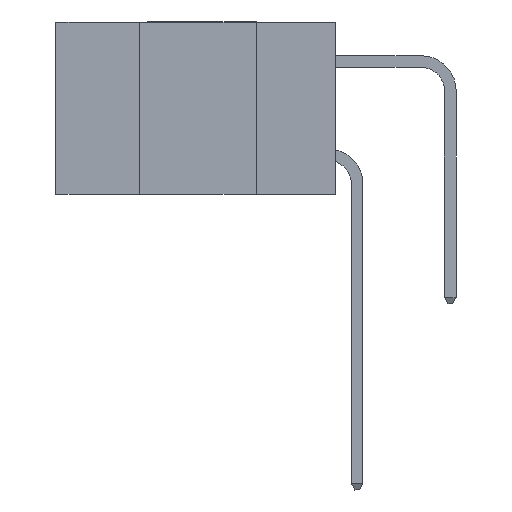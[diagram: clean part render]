
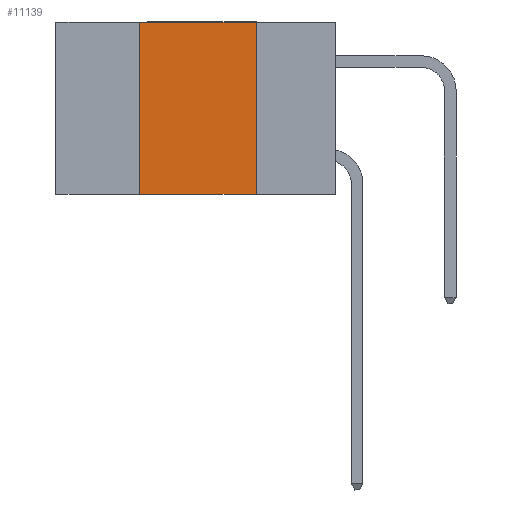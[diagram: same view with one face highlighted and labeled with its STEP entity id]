
A CAD part, left-side view. The second image highlights one B-rep face of the part: STEP entity #11139.
In plain terms, the highlighted planar face has unit normal (-1, 0, 0).
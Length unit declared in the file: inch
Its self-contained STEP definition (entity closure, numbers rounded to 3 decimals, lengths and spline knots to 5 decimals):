
#171 = ORIENTED_EDGE ( 'NONE', *, *, #3334, .F. ) ;
#445 = DIRECTION ( 'NONE',  ( 0., 0., 1. ) ) ;
#1408 = CARTESIAN_POINT ( 'NONE',  ( 0., 0.6, 0. ) ) ;
#2060 = LINE ( 'NONE', #5218, #6798 ) ;
#2243 = LINE ( 'NONE', #3809, #11266 ) ;
#2453 = DIRECTION ( 'NONE',  ( 1., 0., 0. ) ) ;
#2928 = DIRECTION ( 'NONE',  ( 0., -1., 0. ) ) ;
#3334 = EDGE_CURVE ( 'NONE', #9514, #6321, #7796, .T. ) ;
#3809 = CARTESIAN_POINT ( 'NONE',  ( 0., 0.6, -0.37 ) ) ;
#4106 = FACE_OUTER_BOUND ( 'NONE', #6599, .T. ) ;
#4191 = VERTEX_POINT ( 'NONE', #8564 ) ;
#4401 = ORIENTED_EDGE ( 'NONE', *, *, #10520, .F. ) ;
#4851 = CARTESIAN_POINT ( 'NONE',  ( 0., 0.17, -0.37 ) ) ;
#4904 = ORIENTED_EDGE ( 'NONE', *, *, #9249, .F. ) ;
#5218 = CARTESIAN_POINT ( 'NONE',  ( 0., 0.6, 0. ) ) ;
#5571 = CARTESIAN_POINT ( 'NONE',  ( 0., 0.17, 0. ) ) ;
#5963 = EDGE_CURVE ( 'NONE', #8981, #6321, #2243, .T. ) ;
#6321 = VERTEX_POINT ( 'NONE', #4851 ) ;
#6599 = EDGE_LOOP ( 'NONE', ( #171, #4401, #4904, #10034 ) ) ;
#6753 = CARTESIAN_POINT ( 'NONE',  ( 0., 0.42, -0.37 ) ) ;
#6798 = VECTOR ( 'NONE', #7093, 39.37008 ) ;
#7093 = DIRECTION ( 'NONE',  ( 0., -1., 0. ) ) ;
#7796 = LINE ( 'NONE', #5571, #8053 ) ;
#8053 = VECTOR ( 'NONE', #9958, 39.37008 ) ;
#8564 = CARTESIAN_POINT ( 'NONE',  ( 0., 0.42, 0. ) ) ;
#8762 = VECTOR ( 'NONE', #445, 39.37008 ) ;
#8771 = AXIS2_PLACEMENT_3D ( 'NONE', #1408, #2453, #8844 ) ;
#8844 = DIRECTION ( 'NONE',  ( 0., 0., -1. ) ) ;
#8981 = VERTEX_POINT ( 'NONE', #6753 ) ;
#9249 = EDGE_CURVE ( 'NONE', #8981, #4191, #11061, .T. ) ;
#9514 = VERTEX_POINT ( 'NONE', #10010 ) ;
#9661 = CARTESIAN_POINT ( 'NONE',  ( 0., 0.42, 0. ) ) ;
#9958 = DIRECTION ( 'NONE',  ( 0., 0., -1. ) ) ;
#10010 = CARTESIAN_POINT ( 'NONE',  ( 0., 0.17, 0. ) ) ;
#10034 = ORIENTED_EDGE ( 'NONE', *, *, #5963, .T. ) ;
#10520 = EDGE_CURVE ( 'NONE', #4191, #9514, #2060, .T. ) ;
#11061 = LINE ( 'NONE', #9661, #8762 ) ;
#11139 = ADVANCED_FACE ( 'NONE', ( #4106 ), #11402, .F. ) ;
#11266 = VECTOR ( 'NONE', #2928, 39.37008 ) ;
#11402 = PLANE ( 'NONE',  #8771 ) ;
